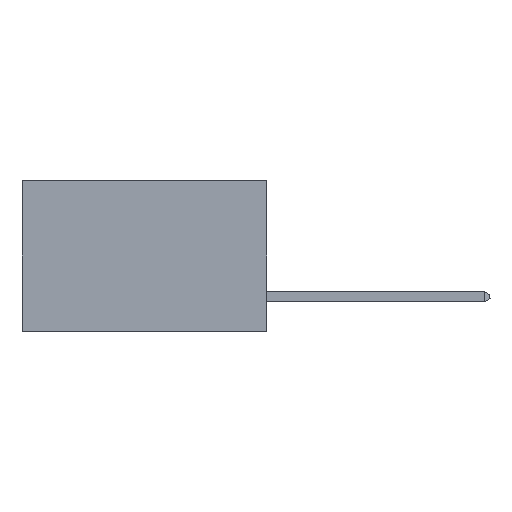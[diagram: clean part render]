
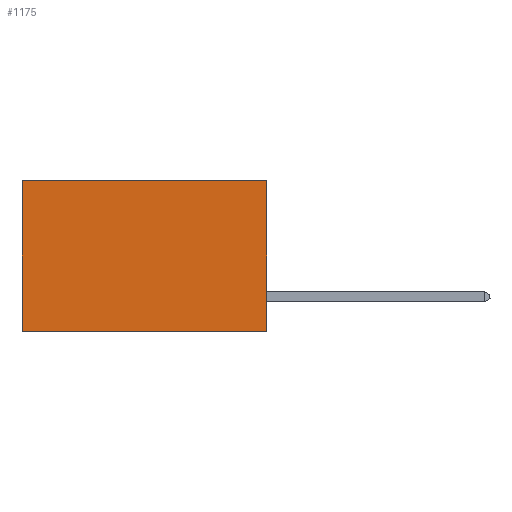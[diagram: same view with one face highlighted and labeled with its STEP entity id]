
A CAD part, left-side view. The second image highlights one B-rep face of the part: STEP entity #1175.
In plain terms, the highlighted planar face has unit normal (-1, 0, 0).
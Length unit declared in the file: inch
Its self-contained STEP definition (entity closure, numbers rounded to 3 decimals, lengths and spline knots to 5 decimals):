
#419 = VERTEX_POINT ( 'NONE', #17405 ) ;
#1175 = ADVANCED_FACE ( 'NONE', ( #9749 ), #12123, .F. ) ;
#1437 = VERTEX_POINT ( 'NONE', #4913 ) ;
#1946 = ORIENTED_EDGE ( 'NONE', *, *, #21557, .F. ) ;
#2022 = VECTOR ( 'NONE', #22296, 39.37008 ) ;
#2530 = CARTESIAN_POINT ( 'NONE',  ( 0.2875, 0., -0.37 ) ) ;
#2932 = VECTOR ( 'NONE', #3465, 39.37008 ) ;
#3465 = DIRECTION ( 'NONE',  ( 0., 0., -1. ) ) ;
#3470 = LINE ( 'NONE', #10427, #13879 ) ;
#4529 = EDGE_CURVE ( 'NONE', #6962, #14830, #4572, .T. ) ;
#4572 = LINE ( 'NONE', #16854, #2022 ) ;
#4683 = CARTESIAN_POINT ( 'NONE',  ( 0.2875, 0.6, 0. ) ) ;
#4913 = CARTESIAN_POINT ( 'NONE',  ( 0.2875, 0., -0.37 ) ) ;
#5218 = CARTESIAN_POINT ( 'NONE',  ( 0.2875, 0., 0. ) ) ;
#5221 = EDGE_LOOP ( 'NONE', ( #20721, #1946, #8692, #20327 ) ) ;
#6257 = DIRECTION ( 'NONE',  ( 1., 0., 0. ) ) ;
#6962 = VERTEX_POINT ( 'NONE', #4683 ) ;
#7090 = AXIS2_PLACEMENT_3D ( 'NONE', #17700, #6257, #10081 ) ;
#8134 = DIRECTION ( 'NONE',  ( 0., 1., 0. ) ) ;
#8340 = VECTOR ( 'NONE', #8134, 39.37008 ) ;
#8692 = ORIENTED_EDGE ( 'NONE', *, *, #13517, .F. ) ;
#9749 = FACE_OUTER_BOUND ( 'NONE', #5221, .T. ) ;
#10081 = DIRECTION ( 'NONE',  ( 0., 0., -1. ) ) ;
#10427 = CARTESIAN_POINT ( 'NONE',  ( 0.2875, 0., 0. ) ) ;
#12123 = PLANE ( 'NONE',  #7090 ) ;
#13517 = EDGE_CURVE ( 'NONE', #419, #1437, #17376, .T. ) ;
#13879 = VECTOR ( 'NONE', #15913, 39.37008 ) ;
#14062 = EDGE_CURVE ( 'NONE', #419, #6962, #3470, .T. ) ;
#14830 = VERTEX_POINT ( 'NONE', #17807 ) ;
#15913 = DIRECTION ( 'NONE',  ( 0., 1., 0. ) ) ;
#16854 = CARTESIAN_POINT ( 'NONE',  ( 0.2875, 0.6, 0. ) ) ;
#17376 = LINE ( 'NONE', #5218, #2932 ) ;
#17405 = CARTESIAN_POINT ( 'NONE',  ( 0.2875, 0., 0. ) ) ;
#17700 = CARTESIAN_POINT ( 'NONE',  ( 0.2875, 0., 0. ) ) ;
#17807 = CARTESIAN_POINT ( 'NONE',  ( 0.2875, 0.6, -0.37 ) ) ;
#20327 = ORIENTED_EDGE ( 'NONE', *, *, #14062, .T. ) ;
#20721 = ORIENTED_EDGE ( 'NONE', *, *, #4529, .T. ) ;
#21103 = LINE ( 'NONE', #2530, #8340 ) ;
#21557 = EDGE_CURVE ( 'NONE', #1437, #14830, #21103, .T. ) ;
#22296 = DIRECTION ( 'NONE',  ( 0., 0., -1. ) ) ;
